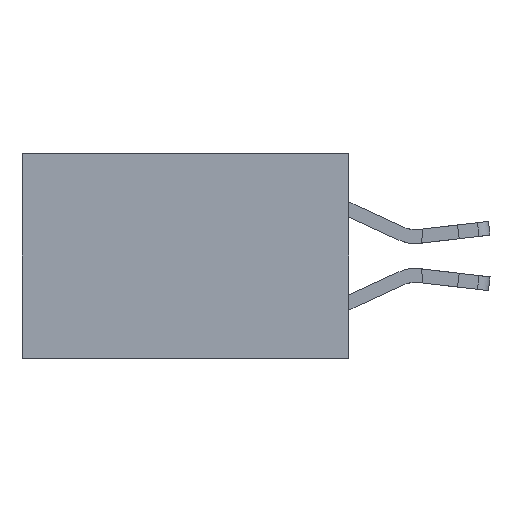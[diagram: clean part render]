
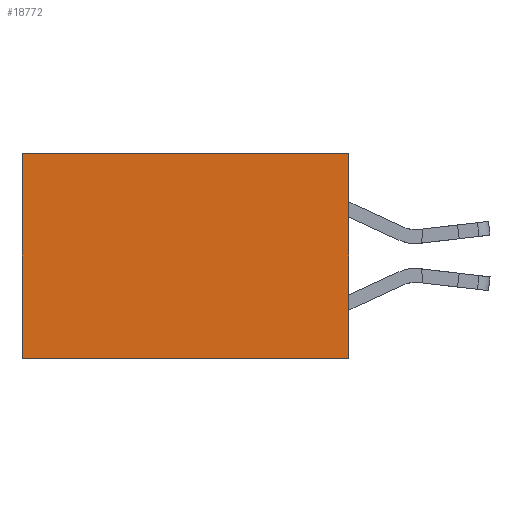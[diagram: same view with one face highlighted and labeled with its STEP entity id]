
A CAD part, left-side view. The second image highlights one B-rep face of the part: STEP entity #18772.
In plain terms, the highlighted planar face has unit normal (-1, 0, 0).
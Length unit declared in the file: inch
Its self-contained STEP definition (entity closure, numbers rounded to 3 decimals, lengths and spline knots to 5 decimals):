
#398 = ORIENTED_EDGE ( 'NONE', *, *, #16102, .F. ) ;
#1341 = EDGE_LOOP ( 'NONE', ( #19810, #398, #4669, #6710 ) ) ;
#1385 = CARTESIAN_POINT ( 'NONE',  ( 0.277, 0., -0.37 ) ) ;
#2717 = VERTEX_POINT ( 'NONE', #14838 ) ;
#3114 = DIRECTION ( 'NONE',  ( 0., 1., 0. ) ) ;
#3272 = LINE ( 'NONE', #18142, #7095 ) ;
#4092 = CARTESIAN_POINT ( 'NONE',  ( 0.277, 0., 0. ) ) ;
#4669 = ORIENTED_EDGE ( 'NONE', *, *, #19821, .F. ) ;
#4874 = DIRECTION ( 'NONE',  ( 1., 0., 0. ) ) ;
#5929 = CARTESIAN_POINT ( 'NONE',  ( 0.277, 0.59, -0.37 ) ) ;
#6608 = LINE ( 'NONE', #13359, #10781 ) ;
#6710 = ORIENTED_EDGE ( 'NONE', *, *, #9082, .T. ) ;
#7095 = VECTOR ( 'NONE', #16575, 39.37008 ) ;
#7214 = AXIS2_PLACEMENT_3D ( 'NONE', #18866, #4874, #15849 ) ;
#8084 = CARTESIAN_POINT ( 'NONE',  ( 0.277, 0.59, 0. ) ) ;
#8436 = VECTOR ( 'NONE', #9926, 39.37008 ) ;
#9082 = EDGE_CURVE ( 'NONE', #13875, #11055, #16728, .T. ) ;
#9780 = VECTOR ( 'NONE', #3114, 39.37008 ) ;
#9926 = DIRECTION ( 'NONE',  ( 0., 1., 0. ) ) ;
#9968 = CARTESIAN_POINT ( 'NONE',  ( 0.277, 0., 0. ) ) ;
#10781 = VECTOR ( 'NONE', #19560, 39.37008 ) ;
#11055 = VERTEX_POINT ( 'NONE', #8084 ) ;
#11183 = VERTEX_POINT ( 'NONE', #5929 ) ;
#11259 = FACE_OUTER_BOUND ( 'NONE', #1341, .T. ) ;
#13359 = CARTESIAN_POINT ( 'NONE',  ( 0.277, 0.59, -0.37 ) ) ;
#13875 = VERTEX_POINT ( 'NONE', #4092 ) ;
#14284 = PLANE ( 'NONE',  #7214 ) ;
#14838 = CARTESIAN_POINT ( 'NONE',  ( 0.277, 0., -0.37 ) ) ;
#15849 = DIRECTION ( 'NONE',  ( 0., 0., -1. ) ) ;
#16102 = EDGE_CURVE ( 'NONE', #2717, #11183, #18042, .T. ) ;
#16575 = DIRECTION ( 'NONE',  ( 0., 0., -1. ) ) ;
#16728 = LINE ( 'NONE', #9968, #8436 ) ;
#18042 = LINE ( 'NONE', #1385, #9780 ) ;
#18142 = CARTESIAN_POINT ( 'NONE',  ( 0.277, 0., -0.37 ) ) ;
#18363 = EDGE_CURVE ( 'NONE', #11055, #11183, #6608, .T. ) ;
#18772 = ADVANCED_FACE ( 'NONE', ( #11259 ), #14284, .F. ) ;
#18866 = CARTESIAN_POINT ( 'NONE',  ( 0.277, 0., -0.37 ) ) ;
#19560 = DIRECTION ( 'NONE',  ( 0., 0., -1. ) ) ;
#19810 = ORIENTED_EDGE ( 'NONE', *, *, #18363, .T. ) ;
#19821 = EDGE_CURVE ( 'NONE', #13875, #2717, #3272, .T. ) ;
